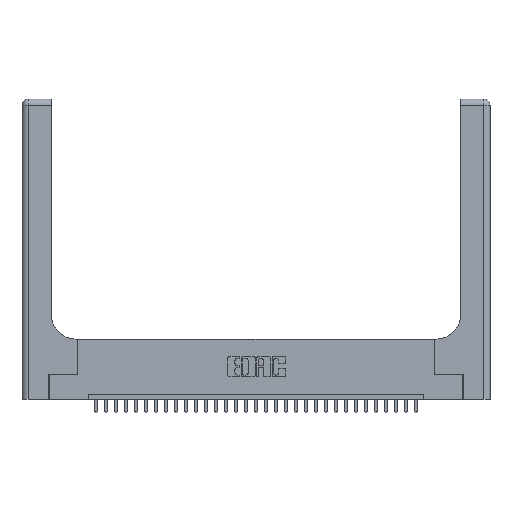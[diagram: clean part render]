
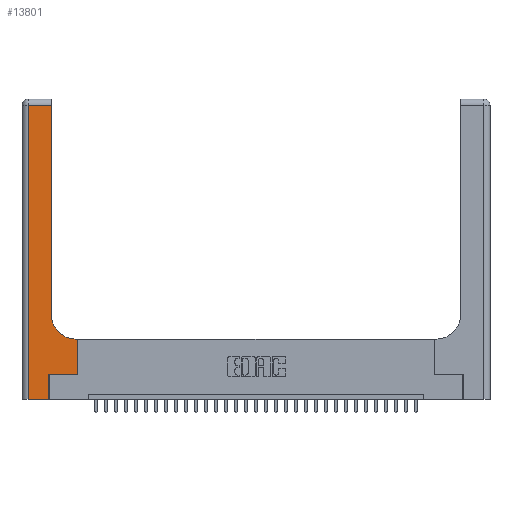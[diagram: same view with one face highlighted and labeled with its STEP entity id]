
A CAD part, top view. The second image highlights one B-rep face of the part: STEP entity #13801.
In plain terms, the highlighted planar face has unit normal (0, 0, 1).
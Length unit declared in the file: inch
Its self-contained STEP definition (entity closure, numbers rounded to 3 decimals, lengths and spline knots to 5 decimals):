
#1558 = EDGE_CURVE ( 'NONE', #22089, #17417, #5679, .T. ) ;
#1607 = VECTOR ( 'NONE', #20309, 39.37008 ) ;
#1783 = EDGE_CURVE ( 'NONE', #17580, #21223, #17769, .T. ) ;
#3234 = CARTESIAN_POINT ( 'NONE',  ( 0., 0., 0.37 ) ) ;
#3781 = DIRECTION ( 'NONE',  ( -1., 0., 0. ) ) ;
#3917 = FACE_OUTER_BOUND ( 'NONE', #12217, .T. ) ;
#4356 = ORIENTED_EDGE ( 'NONE', *, *, #15435, .T. ) ;
#5264 = VECTOR ( 'NONE', #3781, 39.37008 ) ;
#5679 = LINE ( 'NONE', #7197, #10196 ) ;
#7197 = CARTESIAN_POINT ( 'NONE',  ( 0.5585, 0.25, 0.37 ) ) ;
#7954 = DIRECTION ( 'NONE',  ( 1., 0., 0. ) ) ;
#8014 = LINE ( 'NONE', #28155, #8744 ) ;
#8208 = CARTESIAN_POINT ( 'NONE',  ( 0.5415, 0.85, 0.37 ) ) ;
#8227 = EDGE_CURVE ( 'NONE', #17417, #17212, #8014, .T. ) ;
#8532 = DIRECTION ( 'NONE',  ( 0., 0., -1. ) ) ;
#8744 = VECTOR ( 'NONE', #30366, 39.37008 ) ;
#9319 = ORIENTED_EDGE ( 'NONE', *, *, #10660, .T. ) ;
#9779 = CARTESIAN_POINT ( 'NONE',  ( 0.269, 0., 0.37 ) ) ;
#9956 = CARTESIAN_POINT ( 'NONE',  ( 0.2915, 0.85, 0.37 ) ) ;
#10196 = VECTOR ( 'NONE', #14677, 39.37008 ) ;
#10660 = EDGE_CURVE ( 'NONE', #26941, #17580, #26438, .T. ) ;
#10876 = EDGE_CURVE ( 'NONE', #21223, #20312, #16205, .T. ) ;
#11876 = ORIENTED_EDGE ( 'NONE', *, *, #10876, .T. ) ;
#12217 = EDGE_LOOP ( 'NONE', ( #9319, #15978, #11876, #15384, #4356, #27384, #29610, #30316, #23189 ) ) ;
#12463 = EDGE_CURVE ( 'NONE', #17212, #26941, #17243, .T. ) ;
#13801 = ADVANCED_FACE ( 'NONE', ( #3917 ), #25336, .F. ) ;
#14677 = DIRECTION ( 'NONE',  ( 0., 1., 0. ) ) ;
#14694 = CARTESIAN_POINT ( 'NONE',  ( 0.5585, 0.6, 0.37 ) ) ;
#14705 = VECTOR ( 'NONE', #27326, 39.37008 ) ;
#15162 = EDGE_CURVE ( 'NONE', #20312, #18688, #28843, .T. ) ;
#15384 = ORIENTED_EDGE ( 'NONE', *, *, #15162, .T. ) ;
#15435 = EDGE_CURVE ( 'NONE', #18688, #29213, #25766, .T. ) ;
#15457 = VECTOR ( 'NONE', #31011, 39.37008 ) ;
#15978 = ORIENTED_EDGE ( 'NONE', *, *, #1783, .T. ) ;
#15986 = CARTESIAN_POINT ( 'NONE',  ( 0.06, 2.94, 0.37 ) ) ;
#16205 = LINE ( 'NONE', #24899, #14705 ) ;
#16649 = CARTESIAN_POINT ( 'NONE',  ( 0.2915, 3., 0.37 ) ) ;
#17212 = VERTEX_POINT ( 'NONE', #30963 ) ;
#17243 = CIRCLE ( 'NONE', #17434, 0.25 ) ;
#17417 = VERTEX_POINT ( 'NONE', #14694 ) ;
#17434 = AXIS2_PLACEMENT_3D ( 'NONE', #8208, #22830, #30159 ) ;
#17580 = VERTEX_POINT ( 'NONE', #17752 ) ;
#17696 = DIRECTION ( 'NONE',  ( 0., 1., 0. ) ) ;
#17752 = CARTESIAN_POINT ( 'NONE',  ( 0.2915, 2.94, 0.37 ) ) ;
#17769 = LINE ( 'NONE', #25427, #5264 ) ;
#18004 = CARTESIAN_POINT ( 'NONE',  ( 0.269, 0., 0.37 ) ) ;
#18236 = DIRECTION ( 'NONE',  ( -1., 0., 0. ) ) ;
#18556 = CARTESIAN_POINT ( 'NONE',  ( 0.269, 0.25, 0.37 ) ) ;
#18688 = VERTEX_POINT ( 'NONE', #9779 ) ;
#19271 = VECTOR ( 'NONE', #7954, 39.37008 ) ;
#19901 = AXIS2_PLACEMENT_3D ( 'NONE', #27763, #8532, #18236 ) ;
#20309 = DIRECTION ( 'NONE',  ( 1., 0., 0. ) ) ;
#20312 = VERTEX_POINT ( 'NONE', #22046 ) ;
#20741 = LINE ( 'NONE', #26852, #19271 ) ;
#20817 = VECTOR ( 'NONE', #17696, 39.37008 ) ;
#21223 = VERTEX_POINT ( 'NONE', #15986 ) ;
#22046 = CARTESIAN_POINT ( 'NONE',  ( 0.06, 0., 0.37 ) ) ;
#22089 = VERTEX_POINT ( 'NONE', #24042 ) ;
#22830 = DIRECTION ( 'NONE',  ( 0., 0., -1. ) ) ;
#23189 = ORIENTED_EDGE ( 'NONE', *, *, #12463, .T. ) ;
#24042 = CARTESIAN_POINT ( 'NONE',  ( 0.5585, 0.25, 0.37 ) ) ;
#24899 = CARTESIAN_POINT ( 'NONE',  ( 0.06, 3., 0.37 ) ) ;
#25336 = PLANE ( 'NONE',  #19901 ) ;
#25427 = CARTESIAN_POINT ( 'NONE',  ( 0., 2.94, 0.37 ) ) ;
#25766 = LINE ( 'NONE', #18004, #20817 ) ;
#26438 = LINE ( 'NONE', #16649, #15457 ) ;
#26852 = CARTESIAN_POINT ( 'NONE',  ( 0.269, 0.25, 0.37 ) ) ;
#26941 = VERTEX_POINT ( 'NONE', #9956 ) ;
#27326 = DIRECTION ( 'NONE',  ( 0., -1., 0. ) ) ;
#27384 = ORIENTED_EDGE ( 'NONE', *, *, #28525, .T. ) ;
#27763 = CARTESIAN_POINT ( 'NONE',  ( 0., 3., 0.37 ) ) ;
#28155 = CARTESIAN_POINT ( 'NONE',  ( 0.2915, 0.6, 0.37 ) ) ;
#28525 = EDGE_CURVE ( 'NONE', #29213, #22089, #20741, .T. ) ;
#28843 = LINE ( 'NONE', #3234, #1607 ) ;
#29213 = VERTEX_POINT ( 'NONE', #18556 ) ;
#29610 = ORIENTED_EDGE ( 'NONE', *, *, #1558, .T. ) ;
#30159 = DIRECTION ( 'NONE',  ( 1., 0., 0. ) ) ;
#30316 = ORIENTED_EDGE ( 'NONE', *, *, #8227, .T. ) ;
#30366 = DIRECTION ( 'NONE',  ( -1., 0., 0. ) ) ;
#30963 = CARTESIAN_POINT ( 'NONE',  ( 0.5415, 0.6, 0.37 ) ) ;
#31011 = DIRECTION ( 'NONE',  ( 0., 1., 0. ) ) ;
